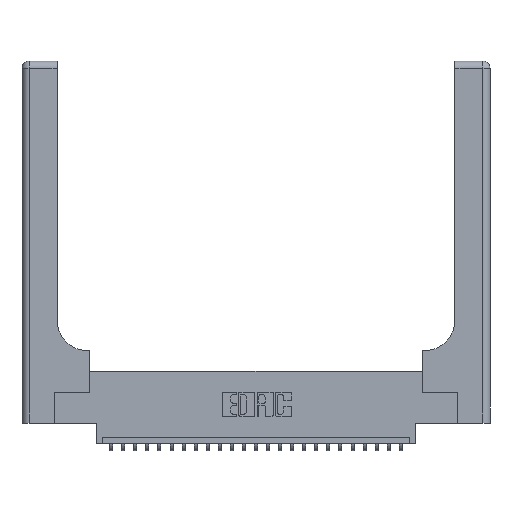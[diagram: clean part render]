
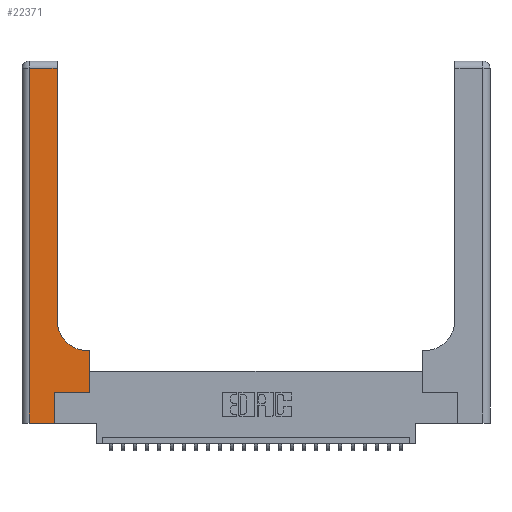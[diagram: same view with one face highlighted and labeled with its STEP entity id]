
A CAD part, top view. The second image highlights one B-rep face of the part: STEP entity #22371.
In plain terms, the highlighted planar face has unit normal (0, 0, 1).
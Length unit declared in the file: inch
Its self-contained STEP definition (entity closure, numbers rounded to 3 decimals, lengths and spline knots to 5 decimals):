
#177 = VERTEX_POINT ( 'NONE', #14864 ) ;
#3287 = CARTESIAN_POINT ( 'NONE',  ( 0.06, 0., 0.37 ) ) ;
#3852 = DIRECTION ( 'NONE',  ( 0., 0., -1. ) ) ;
#4573 = VERTEX_POINT ( 'NONE', #15231 ) ;
#4590 = EDGE_CURVE ( 'NONE', #18630, #15979, #16448, .T. ) ;
#4708 = AXIS2_PLACEMENT_3D ( 'NONE', #12235, #18224, #8276 ) ;
#4896 = LINE ( 'NONE', #11728, #11265 ) ;
#4915 = DIRECTION ( 'NONE',  ( 0., 1., 0. ) ) ;
#5291 = DIRECTION ( 'NONE',  ( 1., 0., 0. ) ) ;
#5618 = EDGE_LOOP ( 'NONE', ( #23037, #26385, #18311, #16974, #22749, #6940, #15949, #18852, #18226 ) ) ;
#5824 = VERTEX_POINT ( 'NONE', #7458 ) ;
#5842 = VECTOR ( 'NONE', #5291, 39.37008 ) ;
#5919 = EDGE_CURVE ( 'NONE', #16185, #14982, #13287, .T. ) ;
#6106 = EDGE_CURVE ( 'NONE', #14982, #8851, #20914, .T. ) ;
#6940 = ORIENTED_EDGE ( 'NONE', *, *, #17278, .T. ) ;
#7185 = CARTESIAN_POINT ( 'NONE',  ( 0.5585, 0.6, 0.37 ) ) ;
#7458 = CARTESIAN_POINT ( 'NONE',  ( 0.5585, 0.25, 0.37 ) ) ;
#7939 = VECTOR ( 'NONE', #4915, 39.37008 ) ;
#8276 = DIRECTION ( 'NONE',  ( 1., 0., 0. ) ) ;
#8280 = CARTESIAN_POINT ( 'NONE',  ( 0., 3., 0.37 ) ) ;
#8541 = DIRECTION ( 'NONE',  ( 0., 1., 0. ) ) ;
#8758 = CARTESIAN_POINT ( 'NONE',  ( 0.5585, 0.25, 0.37 ) ) ;
#8836 = EDGE_CURVE ( 'NONE', #5824, #18630, #9281, .T. ) ;
#8851 = VERTEX_POINT ( 'NONE', #18970 ) ;
#8901 = CARTESIAN_POINT ( 'NONE',  ( 0., 0., 0.37 ) ) ;
#9281 = LINE ( 'NONE', #8758, #19450 ) ;
#9781 = VECTOR ( 'NONE', #15117, 39.37008 ) ;
#10305 = PLANE ( 'NONE',  #22762 ) ;
#10609 = CARTESIAN_POINT ( 'NONE',  ( 0., 2.94, 0.37 ) ) ;
#11265 = VECTOR ( 'NONE', #26021, 39.37008 ) ;
#11728 = CARTESIAN_POINT ( 'NONE',  ( 0.06, 3., 0.37 ) ) ;
#12235 = CARTESIAN_POINT ( 'NONE',  ( 0.5415, 0.85, 0.37 ) ) ;
#12239 = DIRECTION ( 'NONE',  ( -1., 0., 0. ) ) ;
#12493 = EDGE_CURVE ( 'NONE', #15979, #16185, #13550, .T. ) ;
#12968 = DIRECTION ( 'NONE',  ( 1., 0., 0. ) ) ;
#13042 = CARTESIAN_POINT ( 'NONE',  ( 0.2915, 2.94, 0.37 ) ) ;
#13287 = LINE ( 'NONE', #25113, #25135 ) ;
#13536 = EDGE_CURVE ( 'NONE', #8851, #14990, #4896, .T. ) ;
#13550 = CIRCLE ( 'NONE', #4708, 0.25 ) ;
#14250 = LINE ( 'NONE', #18809, #7939 ) ;
#14825 = LINE ( 'NONE', #8901, #15780 ) ;
#14864 = CARTESIAN_POINT ( 'NONE',  ( 0.269, 0.25, 0.37 ) ) ;
#14951 = DIRECTION ( 'NONE',  ( 0., 1., 0. ) ) ;
#14982 = VERTEX_POINT ( 'NONE', #13042 ) ;
#14990 = VERTEX_POINT ( 'NONE', #3287 ) ;
#15117 = DIRECTION ( 'NONE',  ( -1., 0., 0. ) ) ;
#15231 = CARTESIAN_POINT ( 'NONE',  ( 0.269, 0., 0.37 ) ) ;
#15437 = EDGE_CURVE ( 'NONE', #14990, #4573, #14825, .T. ) ;
#15780 = VECTOR ( 'NONE', #12968, 39.37008 ) ;
#15949 = ORIENTED_EDGE ( 'NONE', *, *, #8836, .T. ) ;
#15979 = VERTEX_POINT ( 'NONE', #20065 ) ;
#16185 = VERTEX_POINT ( 'NONE', #19631 ) ;
#16448 = LINE ( 'NONE', #25340, #23814 ) ;
#16974 = ORIENTED_EDGE ( 'NONE', *, *, #15437, .T. ) ;
#17278 = EDGE_CURVE ( 'NONE', #177, #5824, #20766, .T. ) ;
#17486 = CARTESIAN_POINT ( 'NONE',  ( 0.269, 0.25, 0.37 ) ) ;
#18224 = DIRECTION ( 'NONE',  ( 0., 0., -1. ) ) ;
#18226 = ORIENTED_EDGE ( 'NONE', *, *, #12493, .T. ) ;
#18311 = ORIENTED_EDGE ( 'NONE', *, *, #13536, .T. ) ;
#18630 = VERTEX_POINT ( 'NONE', #7185 ) ;
#18809 = CARTESIAN_POINT ( 'NONE',  ( 0.269, 0., 0.37 ) ) ;
#18852 = ORIENTED_EDGE ( 'NONE', *, *, #4590, .T. ) ;
#18970 = CARTESIAN_POINT ( 'NONE',  ( 0.06, 2.94, 0.37 ) ) ;
#19450 = VECTOR ( 'NONE', #14951, 39.37008 ) ;
#19631 = CARTESIAN_POINT ( 'NONE',  ( 0.2915, 0.85, 0.37 ) ) ;
#20065 = CARTESIAN_POINT ( 'NONE',  ( 0.5415, 0.6, 0.37 ) ) ;
#20766 = LINE ( 'NONE', #17486, #5842 ) ;
#20914 = LINE ( 'NONE', #10609, #9781 ) ;
#21216 = EDGE_CURVE ( 'NONE', #4573, #177, #14250, .T. ) ;
#21527 = FACE_OUTER_BOUND ( 'NONE', #5618, .T. ) ;
#22371 = ADVANCED_FACE ( 'NONE', ( #21527 ), #10305, .F. ) ;
#22749 = ORIENTED_EDGE ( 'NONE', *, *, #21216, .T. ) ;
#22762 = AXIS2_PLACEMENT_3D ( 'NONE', #8280, #3852, #12239 ) ;
#23037 = ORIENTED_EDGE ( 'NONE', *, *, #5919, .T. ) ;
#23270 = DIRECTION ( 'NONE',  ( -1., 0., 0. ) ) ;
#23814 = VECTOR ( 'NONE', #23270, 39.37008 ) ;
#25113 = CARTESIAN_POINT ( 'NONE',  ( 0.2915, 3., 0.37 ) ) ;
#25135 = VECTOR ( 'NONE', #8541, 39.37008 ) ;
#25340 = CARTESIAN_POINT ( 'NONE',  ( 0.2915, 0.6, 0.37 ) ) ;
#26021 = DIRECTION ( 'NONE',  ( 0., -1., 0. ) ) ;
#26385 = ORIENTED_EDGE ( 'NONE', *, *, #6106, .T. ) ;
